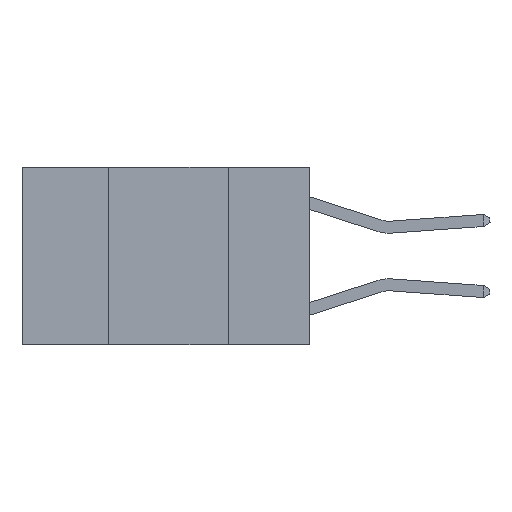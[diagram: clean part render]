
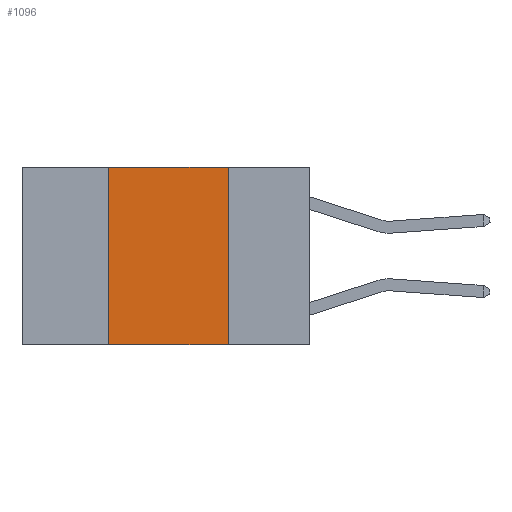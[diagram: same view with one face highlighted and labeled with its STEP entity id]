
A CAD part, left-side view. The second image highlights one B-rep face of the part: STEP entity #1096.
In plain terms, the highlighted planar face has unit normal (-1, 0, 0).
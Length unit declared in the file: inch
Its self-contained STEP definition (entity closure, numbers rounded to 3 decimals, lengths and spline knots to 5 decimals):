
#550 = EDGE_CURVE ( 'NONE', #2186, #1377, #2072, .T. ) ;
#1017 = LINE ( 'NONE', #1575, #4359 ) ;
#1096 = ADVANCED_FACE ( 'NONE', ( #7253 ), #4507, .F. ) ;
#1224 = EDGE_CURVE ( 'NONE', #1328, #2186, #7583, .T. ) ;
#1328 = VERTEX_POINT ( 'NONE', #2107 ) ;
#1377 = VERTEX_POINT ( 'NONE', #5576 ) ;
#1575 = CARTESIAN_POINT ( 'NONE',  ( 0., 0.17, 0. ) ) ;
#1585 = AXIS2_PLACEMENT_3D ( 'NONE', #4688, #7702, #7501 ) ;
#2044 = DIRECTION ( 'NONE',  ( 0., -1., 0. ) ) ;
#2072 = LINE ( 'NONE', #5617, #9307 ) ;
#2107 = CARTESIAN_POINT ( 'NONE',  ( 0., 0.42, -0.37 ) ) ;
#2186 = VERTEX_POINT ( 'NONE', #8996 ) ;
#2841 = LINE ( 'NONE', #7202, #6176 ) ;
#2928 = ORIENTED_EDGE ( 'NONE', *, *, #3203, .F. ) ;
#3143 = ORIENTED_EDGE ( 'NONE', *, *, #1224, .F. ) ;
#3203 = EDGE_CURVE ( 'NONE', #1377, #8799, #1017, .T. ) ;
#3703 = DIRECTION ( 'NONE',  ( 0., -1., 0. ) ) ;
#3860 = VECTOR ( 'NONE', #7522, 39.37008 ) ;
#4359 = VECTOR ( 'NONE', #8929, 39.37008 ) ;
#4507 = PLANE ( 'NONE',  #1585 ) ;
#4596 = EDGE_LOOP ( 'NONE', ( #2928, #6262, #3143, #8396 ) ) ;
#4688 = CARTESIAN_POINT ( 'NONE',  ( 0., 0.6, 0. ) ) ;
#5542 = CARTESIAN_POINT ( 'NONE',  ( 0., 0.42, 0. ) ) ;
#5576 = CARTESIAN_POINT ( 'NONE',  ( 0., 0.17, 0. ) ) ;
#5591 = CARTESIAN_POINT ( 'NONE',  ( 0., 0.17, -0.37 ) ) ;
#5617 = CARTESIAN_POINT ( 'NONE',  ( 0., 0.6, 0. ) ) ;
#6176 = VECTOR ( 'NONE', #3703, 39.37008 ) ;
#6262 = ORIENTED_EDGE ( 'NONE', *, *, #550, .F. ) ;
#7202 = CARTESIAN_POINT ( 'NONE',  ( 0., 0.6, -0.37 ) ) ;
#7253 = FACE_OUTER_BOUND ( 'NONE', #4596, .T. ) ;
#7501 = DIRECTION ( 'NONE',  ( 0., 0., -1. ) ) ;
#7522 = DIRECTION ( 'NONE',  ( 0., 0., 1. ) ) ;
#7583 = LINE ( 'NONE', #5542, #3860 ) ;
#7702 = DIRECTION ( 'NONE',  ( 1., 0., 0. ) ) ;
#8317 = EDGE_CURVE ( 'NONE', #1328, #8799, #2841, .T. ) ;
#8396 = ORIENTED_EDGE ( 'NONE', *, *, #8317, .T. ) ;
#8799 = VERTEX_POINT ( 'NONE', #5591 ) ;
#8929 = DIRECTION ( 'NONE',  ( 0., 0., -1. ) ) ;
#8996 = CARTESIAN_POINT ( 'NONE',  ( 0., 0.42, 0. ) ) ;
#9307 = VECTOR ( 'NONE', #2044, 39.37008 ) ;
